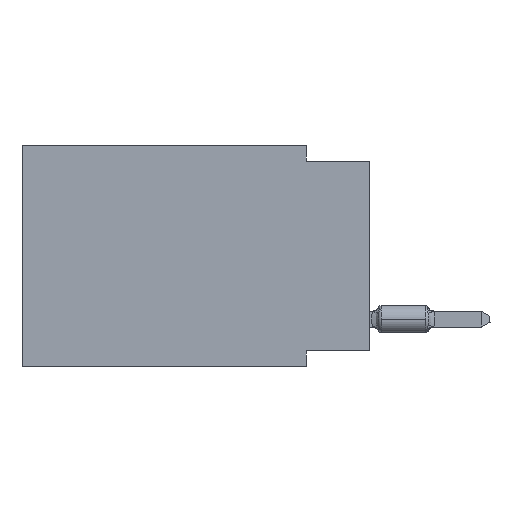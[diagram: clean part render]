
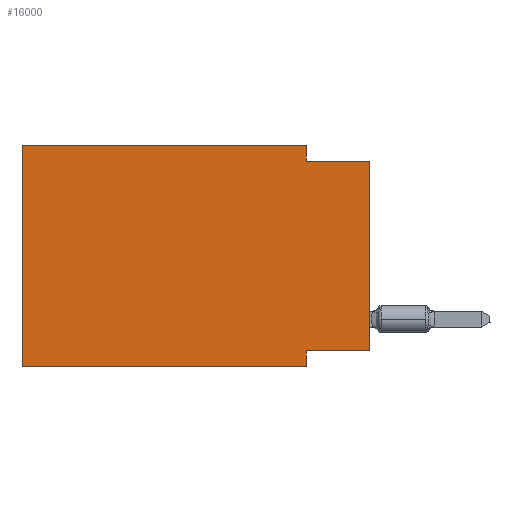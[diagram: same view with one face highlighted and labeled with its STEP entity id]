
A CAD part, left-side view. The second image highlights one B-rep face of the part: STEP entity #16000.
In plain terms, the highlighted planar face has unit normal (-1, 0, 0).
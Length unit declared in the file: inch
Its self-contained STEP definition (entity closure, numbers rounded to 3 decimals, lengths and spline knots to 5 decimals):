
#633 = VECTOR ( 'NONE', #6929, 39.37008 ) ;
#793 = DIRECTION ( 'NONE',  ( 0., 1., 0. ) ) ;
#1977 = LINE ( 'NONE', #56132, #16315 ) ;
#4250 = EDGE_CURVE ( 'NONE', #6222, #38910, #60082, .T. ) ;
#4656 = ORIENTED_EDGE ( 'NONE', *, *, #4250, .T. ) ;
#5342 = PLANE ( 'NONE',  #19222 ) ;
#6222 = VERTEX_POINT ( 'NONE', #75335 ) ;
#6633 = VERTEX_POINT ( 'NONE', #57802 ) ;
#6929 = DIRECTION ( 'NONE',  ( 0., 0., -1. ) ) ;
#10070 = CARTESIAN_POINT ( 'NONE',  ( 0., 0.1, -0.35 ) ) ;
#11018 = EDGE_CURVE ( 'NONE', #38349, #6633, #30722, .T. ) ;
#11861 = ORIENTED_EDGE ( 'NONE', *, *, #63607, .F. ) ;
#13852 = EDGE_CURVE ( 'NONE', #40441, #15420, #1977, .T. ) ;
#14725 = CARTESIAN_POINT ( 'NONE',  ( 0., 0.55, 0. ) ) ;
#15420 = VERTEX_POINT ( 'NONE', #20084 ) ;
#16000 = ADVANCED_FACE ( 'NONE', ( #23122 ), #5342, .F. ) ;
#16315 = VECTOR ( 'NONE', #793, 39.37008 ) ;
#18643 = EDGE_CURVE ( 'NONE', #21116, #47584, #74562, .T. ) ;
#19222 = AXIS2_PLACEMENT_3D ( 'NONE', #36044, #73218, #41705 ) ;
#19395 = LINE ( 'NONE', #57723, #38955 ) ;
#20084 = CARTESIAN_POINT ( 'NONE',  ( 0., 0.1, -0.325 ) ) ;
#20373 = VECTOR ( 'NONE', #64017, 39.37008 ) ;
#21116 = VERTEX_POINT ( 'NONE', #50262 ) ;
#22119 = DIRECTION ( 'NONE',  ( 0., -1., 0. ) ) ;
#23122 = FACE_OUTER_BOUND ( 'NONE', #27627, .T. ) ;
#27474 = ORIENTED_EDGE ( 'NONE', *, *, #11018, .F. ) ;
#27627 = EDGE_LOOP ( 'NONE', ( #42531, #45966, #41284, #27474, #11861, #4656, #31463, #50150 ) ) ;
#28653 = DIRECTION ( 'NONE',  ( 0., 0., -1. ) ) ;
#30722 = LINE ( 'NONE', #49312, #54720 ) ;
#31463 = ORIENTED_EDGE ( 'NONE', *, *, #42625, .F. ) ;
#33918 = LINE ( 'NONE', #10070, #74230 ) ;
#35299 = CARTESIAN_POINT ( 'NONE',  ( 0., 0.55, 0. ) ) ;
#36044 = CARTESIAN_POINT ( 'NONE',  ( 0., 0.55, 0. ) ) ;
#38349 = VERTEX_POINT ( 'NONE', #35299 ) ;
#38910 = VERTEX_POINT ( 'NONE', #50135 ) ;
#38955 = VECTOR ( 'NONE', #56146, 39.37008 ) ;
#40441 = VERTEX_POINT ( 'NONE', #70490 ) ;
#41284 = ORIENTED_EDGE ( 'NONE', *, *, #42306, .F. ) ;
#41705 = DIRECTION ( 'NONE',  ( 0., 0., -1. ) ) ;
#42078 = LINE ( 'NONE', #73601, #633 ) ;
#42306 = EDGE_CURVE ( 'NONE', #6633, #21116, #42078, .T. ) ;
#42531 = ORIENTED_EDGE ( 'NONE', *, *, #59551, .T. ) ;
#42625 = EDGE_CURVE ( 'NONE', #15420, #38910, #33918, .T. ) ;
#43834 = CARTESIAN_POINT ( 'NONE',  ( 0., 0., -0.025 ) ) ;
#45966 = ORIENTED_EDGE ( 'NONE', *, *, #18643, .F. ) ;
#47584 = VERTEX_POINT ( 'NONE', #67100 ) ;
#49312 = CARTESIAN_POINT ( 'NONE',  ( 0., 0.55, 0. ) ) ;
#50135 = CARTESIAN_POINT ( 'NONE',  ( 0., 0.1, -0.35 ) ) ;
#50150 = ORIENTED_EDGE ( 'NONE', *, *, #13852, .F. ) ;
#50262 = CARTESIAN_POINT ( 'NONE',  ( 0., 0.1, -0.025 ) ) ;
#52502 = VECTOR ( 'NONE', #22119, 39.37008 ) ;
#53070 = LINE ( 'NONE', #14725, #20373 ) ;
#54720 = VECTOR ( 'NONE', #56167, 39.37008 ) ;
#56132 = CARTESIAN_POINT ( 'NONE',  ( 0., 0., -0.325 ) ) ;
#56146 = DIRECTION ( 'NONE',  ( 0., 0., 1. ) ) ;
#56167 = DIRECTION ( 'NONE',  ( 0., -1., 0. ) ) ;
#57723 = CARTESIAN_POINT ( 'NONE',  ( 0., 0., 0. ) ) ;
#57802 = CARTESIAN_POINT ( 'NONE',  ( 0., 0.1, 0. ) ) ;
#59551 = EDGE_CURVE ( 'NONE', #40441, #47584, #19395, .T. ) ;
#60082 = LINE ( 'NONE', #66956, #52502 ) ;
#63607 = EDGE_CURVE ( 'NONE', #6222, #38349, #53070, .T. ) ;
#64017 = DIRECTION ( 'NONE',  ( 0., 0., 1. ) ) ;
#65740 = VECTOR ( 'NONE', #68487, 39.37008 ) ;
#66956 = CARTESIAN_POINT ( 'NONE',  ( 0., 0.55, -0.35 ) ) ;
#67100 = CARTESIAN_POINT ( 'NONE',  ( 0., 0., -0.025 ) ) ;
#68487 = DIRECTION ( 'NONE',  ( 0., -1., 0. ) ) ;
#70490 = CARTESIAN_POINT ( 'NONE',  ( 0., 0., -0.325 ) ) ;
#73218 = DIRECTION ( 'NONE',  ( 1., 0., 0. ) ) ;
#73601 = CARTESIAN_POINT ( 'NONE',  ( 0., 0.1, 0. ) ) ;
#74230 = VECTOR ( 'NONE', #28653, 39.37008 ) ;
#74562 = LINE ( 'NONE', #43834, #65740 ) ;
#75335 = CARTESIAN_POINT ( 'NONE',  ( 0., 0.55, -0.35 ) ) ;
